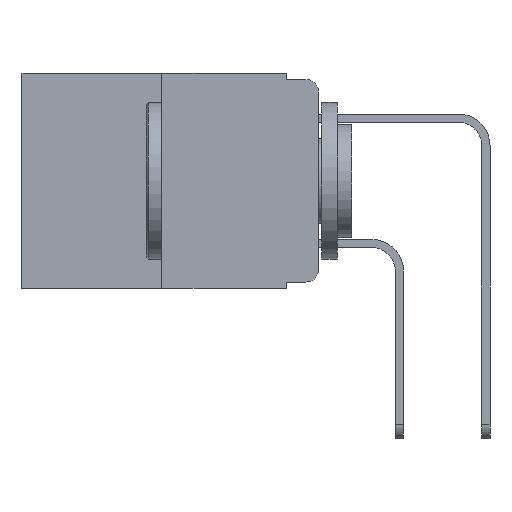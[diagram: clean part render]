
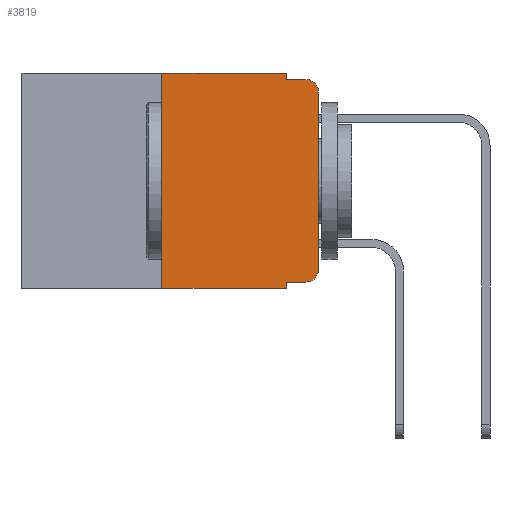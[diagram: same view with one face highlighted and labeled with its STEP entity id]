
A CAD part, left-side view. The second image highlights one B-rep face of the part: STEP entity #3819.
In plain terms, the highlighted planar face has unit normal (-1, 0, 0).
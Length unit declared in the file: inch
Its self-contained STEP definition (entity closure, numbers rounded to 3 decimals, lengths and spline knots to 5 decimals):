
#79 = AXIS2_PLACEMENT_3D ( 'NONE', #5281, #13199, #6467 ) ;
#248 = CARTESIAN_POINT ( 'NONE',  ( 0., 0.02, -0.01 ) ) ;
#647 = EDGE_CURVE ( 'NONE', #4172, #1641, #6779, .T. ) ;
#917 = ORIENTED_EDGE ( 'NONE', *, *, #647, .T. ) ;
#1227 = DIRECTION ( 'NONE',  ( 0., 0., 1. ) ) ;
#1475 = EDGE_CURVE ( 'NONE', #2223, #4172, #2339, .T. ) ;
#1576 = CARTESIAN_POINT ( 'NONE',  ( 0., 0.051, 0. ) ) ;
#1641 = VERTEX_POINT ( 'NONE', #6405 ) ;
#1704 = ORIENTED_EDGE ( 'NONE', *, *, #4648, .F. ) ;
#1749 = VECTOR ( 'NONE', #7045, 39.37008 ) ;
#2223 = VERTEX_POINT ( 'NONE', #14819 ) ;
#2339 = LINE ( 'NONE', #14227, #14479 ) ;
#2383 = DIRECTION ( 'NONE',  ( 0., 0., -1. ) ) ;
#2844 = CIRCLE ( 'NONE', #79, 0.02 ) ;
#2885 = CARTESIAN_POINT ( 'NONE',  ( 0., 0.051, -0.01 ) ) ;
#3061 = EDGE_CURVE ( 'NONE', #2223, #14539, #14459, .T. ) ;
#3292 = CARTESIAN_POINT ( 'NONE',  ( 0., 0.25, -0.343 ) ) ;
#3384 = EDGE_CURVE ( 'NONE', #10759, #10396, #6896, .T. ) ;
#3819 = ADVANCED_FACE ( 'NONE', ( #5140 ), #7881, .F. ) ;
#3851 = EDGE_CURVE ( 'NONE', #11164, #10759, #7897, .T. ) ;
#4031 = CARTESIAN_POINT ( 'NONE',  ( 0., 0.051, -0.343 ) ) ;
#4172 = VERTEX_POINT ( 'NONE', #9643 ) ;
#4204 = EDGE_LOOP ( 'NONE', ( #5791, #6518, #9955, #1704, #8722, #9079, #9793, #10647, #14749, #917 ) ) ;
#4253 = EDGE_CURVE ( 'NONE', #11164, #14539, #5129, .T. ) ;
#4648 = EDGE_CURVE ( 'NONE', #10396, #11518, #11905, .T. ) ;
#5073 = VECTOR ( 'NONE', #2383, 39.37008 ) ;
#5129 = LINE ( 'NONE', #8637, #10880 ) ;
#5140 = FACE_OUTER_BOUND ( 'NONE', #4204, .T. ) ;
#5281 = CARTESIAN_POINT ( 'NONE',  ( 0., 0.02, -0.03 ) ) ;
#5393 = LINE ( 'NONE', #13172, #8131 ) ;
#5458 = EDGE_CURVE ( 'NONE', #11518, #12646, #13960, .T. ) ;
#5791 = ORIENTED_EDGE ( 'NONE', *, *, #7021, .T. ) ;
#5875 = CARTESIAN_POINT ( 'NONE',  ( 0., 0.051, 0. ) ) ;
#5926 = VERTEX_POINT ( 'NONE', #9340 ) ;
#6250 = EDGE_CURVE ( 'NONE', #5926, #12646, #2844, .T. ) ;
#6405 = CARTESIAN_POINT ( 'NONE',  ( 0., 0., -0.313 ) ) ;
#6416 = DIRECTION ( 'NONE',  ( 0., 0., -1. ) ) ;
#6437 = DIRECTION ( 'NONE',  ( -1., 0., 0. ) ) ;
#6464 = CARTESIAN_POINT ( 'NONE',  ( 0., 0.02, -0.313 ) ) ;
#6467 = DIRECTION ( 'NONE',  ( 0., 0., -1. ) ) ;
#6518 = ORIENTED_EDGE ( 'NONE', *, *, #6250, .T. ) ;
#6750 = DIRECTION ( 'NONE',  ( 0., 0., -1. ) ) ;
#6779 = CIRCLE ( 'NONE', #10389, 0.02 ) ;
#6896 = LINE ( 'NONE', #14016, #12539 ) ;
#6977 = CARTESIAN_POINT ( 'NONE',  ( 0., 0.25, 0. ) ) ;
#7021 = EDGE_CURVE ( 'NONE', #1641, #5926, #5393, .T. ) ;
#7034 = DIRECTION ( 'NONE',  ( 0., 0., -1. ) ) ;
#7045 = DIRECTION ( 'NONE',  ( 0., -1., 0. ) ) ;
#7881 = PLANE ( 'NONE',  #12058 ) ;
#7897 = LINE ( 'NONE', #9097, #13482 ) ;
#8131 = VECTOR ( 'NONE', #1227, 39.37008 ) ;
#8637 = CARTESIAN_POINT ( 'NONE',  ( 0., 0.473, -0.343 ) ) ;
#8722 = ORIENTED_EDGE ( 'NONE', *, *, #3384, .F. ) ;
#9079 = ORIENTED_EDGE ( 'NONE', *, *, #3851, .F. ) ;
#9097 = CARTESIAN_POINT ( 'NONE',  ( 0., 0.25, 0. ) ) ;
#9340 = CARTESIAN_POINT ( 'NONE',  ( 0., 0., -0.03 ) ) ;
#9643 = CARTESIAN_POINT ( 'NONE',  ( 0., 0.02, -0.333 ) ) ;
#9793 = ORIENTED_EDGE ( 'NONE', *, *, #4253, .T. ) ;
#9955 = ORIENTED_EDGE ( 'NONE', *, *, #5458, .F. ) ;
#10389 = AXIS2_PLACEMENT_3D ( 'NONE', #6464, #6437, #6416 ) ;
#10396 = VERTEX_POINT ( 'NONE', #12112 ) ;
#10452 = CARTESIAN_POINT ( 'NONE',  ( 0., 0.051, -0.01 ) ) ;
#10647 = ORIENTED_EDGE ( 'NONE', *, *, #3061, .F. ) ;
#10759 = VERTEX_POINT ( 'NONE', #6977 ) ;
#10880 = VECTOR ( 'NONE', #14209, 39.37008 ) ;
#11164 = VERTEX_POINT ( 'NONE', #3292 ) ;
#11257 = CARTESIAN_POINT ( 'NONE',  ( 0., 0.473, 0. ) ) ;
#11303 = DIRECTION ( 'NONE',  ( 0., 0., 1. ) ) ;
#11518 = VERTEX_POINT ( 'NONE', #2885 ) ;
#11905 = LINE ( 'NONE', #5875, #14496 ) ;
#12058 = AXIS2_PLACEMENT_3D ( 'NONE', #11257, #13490, #6750 ) ;
#12112 = CARTESIAN_POINT ( 'NONE',  ( 0., 0.051, 0. ) ) ;
#12539 = VECTOR ( 'NONE', #14040, 39.37008 ) ;
#12646 = VERTEX_POINT ( 'NONE', #248 ) ;
#12707 = DIRECTION ( 'NONE',  ( 0., -1., 0. ) ) ;
#13172 = CARTESIAN_POINT ( 'NONE',  ( 0., 0., 0. ) ) ;
#13199 = DIRECTION ( 'NONE',  ( -1., 0., 0. ) ) ;
#13482 = VECTOR ( 'NONE', #11303, 39.37008 ) ;
#13490 = DIRECTION ( 'NONE',  ( 1., 0., 0. ) ) ;
#13960 = LINE ( 'NONE', #10452, #1749 ) ;
#14016 = CARTESIAN_POINT ( 'NONE',  ( 0., 0.473, 0. ) ) ;
#14040 = DIRECTION ( 'NONE',  ( 0., -1., 0. ) ) ;
#14209 = DIRECTION ( 'NONE',  ( 0., -1., 0. ) ) ;
#14227 = CARTESIAN_POINT ( 'NONE',  ( 0., 0.051, -0.333 ) ) ;
#14459 = LINE ( 'NONE', #1576, #5073 ) ;
#14479 = VECTOR ( 'NONE', #12707, 39.37008 ) ;
#14496 = VECTOR ( 'NONE', #7034, 39.37008 ) ;
#14539 = VERTEX_POINT ( 'NONE', #4031 ) ;
#14749 = ORIENTED_EDGE ( 'NONE', *, *, #1475, .T. ) ;
#14819 = CARTESIAN_POINT ( 'NONE',  ( 0., 0.051, -0.333 ) ) ;
